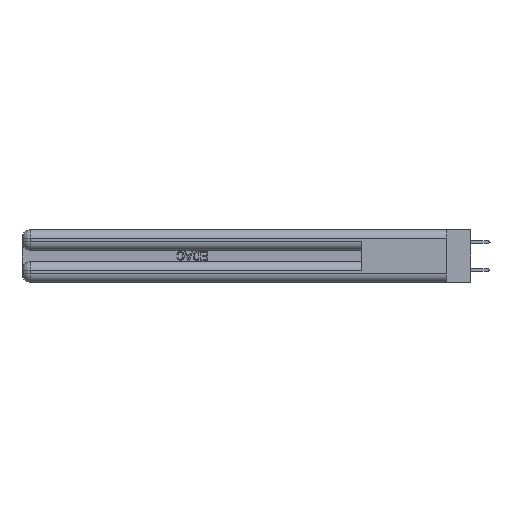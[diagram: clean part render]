
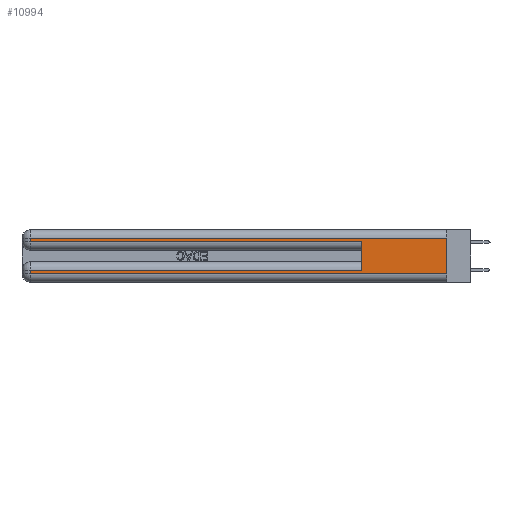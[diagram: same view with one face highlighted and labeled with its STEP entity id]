
A CAD part, left-side view. The second image highlights one B-rep face of the part: STEP entity #10994.
In plain terms, the highlighted planar face has unit normal (-1, 0, 0).
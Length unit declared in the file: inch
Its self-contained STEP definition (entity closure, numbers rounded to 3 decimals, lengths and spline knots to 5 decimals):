
#1044 = VERTEX_POINT ( 'NONE', #24151 ) ;
#1306 = CARTESIAN_POINT ( 'NONE',  ( 0., 0., 0.37 ) ) ;
#1368 = VECTOR ( 'NONE', #18233, 39.37008 ) ;
#1788 = CARTESIAN_POINT ( 'NONE',  ( 0., 2.94, 0.285 ) ) ;
#1818 = VERTEX_POINT ( 'NONE', #13859 ) ;
#2205 = EDGE_CURVE ( 'NONE', #2818, #11704, #24350, .T. ) ;
#2666 = CARTESIAN_POINT ( 'NONE',  ( 0., 0., 0.31 ) ) ;
#2701 = LINE ( 'NONE', #21302, #34925 ) ;
#2818 = VERTEX_POINT ( 'NONE', #1788 ) ;
#4094 = LINE ( 'NONE', #29023, #19522 ) ;
#4219 = CARTESIAN_POINT ( 'NONE',  ( 0., 0.6, 0.085 ) ) ;
#6178 = CARTESIAN_POINT ( 'NONE',  ( 0., 0., 0.06 ) ) ;
#6883 = CARTESIAN_POINT ( 'NONE',  ( 0., 0., 0.06 ) ) ;
#7442 = VECTOR ( 'NONE', #21534, 39.37008 ) ;
#7646 = VECTOR ( 'NONE', #18627, 39.37008 ) ;
#7894 = CARTESIAN_POINT ( 'NONE',  ( 0., 2.94, 0.06 ) ) ;
#7979 = EDGE_CURVE ( 'NONE', #14330, #1818, #37925, .T. ) ;
#8123 = CARTESIAN_POINT ( 'NONE',  ( 0., 0., 0.37 ) ) ;
#8813 = EDGE_CURVE ( 'NONE', #1818, #2818, #15207, .T. ) ;
#9780 = DIRECTION ( 'NONE',  ( 0., 1., 0. ) ) ;
#10994 = ADVANCED_FACE ( 'NONE', ( #35675 ), #36085, .F. ) ;
#11587 = ORIENTED_EDGE ( 'NONE', *, *, #7979, .T. ) ;
#11704 = VERTEX_POINT ( 'NONE', #35297 ) ;
#11729 = DIRECTION ( 'NONE',  ( 0., 1., 0. ) ) ;
#12151 = CARTESIAN_POINT ( 'NONE',  ( 0., 2.94, 0.37 ) ) ;
#12502 = EDGE_CURVE ( 'NONE', #14330, #17520, #14176, .T. ) ;
#12824 = EDGE_CURVE ( 'NONE', #32387, #17520, #24569, .T. ) ;
#13472 = LINE ( 'NONE', #29198, #18146 ) ;
#13502 = DIRECTION ( 'NONE',  ( 0., 0., -1. ) ) ;
#13506 = VECTOR ( 'NONE', #38465, 39.37008 ) ;
#13859 = CARTESIAN_POINT ( 'NONE',  ( 0., 2.94, 0.31 ) ) ;
#14176 = LINE ( 'NONE', #1306, #13506 ) ;
#14330 = VERTEX_POINT ( 'NONE', #2666 ) ;
#14664 = ORIENTED_EDGE ( 'NONE', *, *, #12824, .T. ) ;
#15207 = LINE ( 'NONE', #12151, #7442 ) ;
#15524 = EDGE_CURVE ( 'NONE', #1044, #32387, #4094, .T. ) ;
#16704 = DIRECTION ( 'NONE',  ( 0., 0., -1. ) ) ;
#17295 = ORIENTED_EDGE ( 'NONE', *, *, #15524, .T. ) ;
#17520 = VERTEX_POINT ( 'NONE', #6883 ) ;
#18146 = VECTOR ( 'NONE', #35299, 39.37008 ) ;
#18233 = DIRECTION ( 'NONE',  ( 0., -1., 0. ) ) ;
#18627 = DIRECTION ( 'NONE',  ( 0., -1., 0. ) ) ;
#19522 = VECTOR ( 'NONE', #13502, 39.37008 ) ;
#20545 = ORIENTED_EDGE ( 'NONE', *, *, #2205, .T. ) ;
#21302 = CARTESIAN_POINT ( 'NONE',  ( 0., 0., 0.085 ) ) ;
#21534 = DIRECTION ( 'NONE',  ( 0., 0., -1. ) ) ;
#24048 = ORIENTED_EDGE ( 'NONE', *, *, #12502, .F. ) ;
#24151 = CARTESIAN_POINT ( 'NONE',  ( 0., 2.94, 0.085 ) ) ;
#24350 = LINE ( 'NONE', #36796, #1368 ) ;
#24569 = LINE ( 'NONE', #6178, #7646 ) ;
#27483 = EDGE_CURVE ( 'NONE', #27990, #1044, #2701, .T. ) ;
#27990 = VERTEX_POINT ( 'NONE', #4219 ) ;
#29023 = CARTESIAN_POINT ( 'NONE',  ( 0., 2.94, 0.37 ) ) ;
#29198 = CARTESIAN_POINT ( 'NONE',  ( 0., 0.6, 0.145 ) ) ;
#30406 = EDGE_LOOP ( 'NONE', ( #24048, #11587, #31213, #20545, #34841, #36443, #17295, #14664 ) ) ;
#31213 = ORIENTED_EDGE ( 'NONE', *, *, #8813, .T. ) ;
#31885 = EDGE_CURVE ( 'NONE', #27990, #11704, #13472, .T. ) ;
#32220 = DIRECTION ( 'NONE',  ( 1., 0., 0. ) ) ;
#32387 = VERTEX_POINT ( 'NONE', #7894 ) ;
#34841 = ORIENTED_EDGE ( 'NONE', *, *, #31885, .F. ) ;
#34925 = VECTOR ( 'NONE', #11729, 39.37008 ) ;
#35297 = CARTESIAN_POINT ( 'NONE',  ( 0., 0.6, 0.285 ) ) ;
#35299 = DIRECTION ( 'NONE',  ( 0., 0., 1. ) ) ;
#35675 = FACE_OUTER_BOUND ( 'NONE', #30406, .T. ) ;
#36085 = PLANE ( 'NONE',  #40152 ) ;
#36443 = ORIENTED_EDGE ( 'NONE', *, *, #27483, .T. ) ;
#36796 = CARTESIAN_POINT ( 'NONE',  ( 0., 0., 0.285 ) ) ;
#36813 = VECTOR ( 'NONE', #9780, 39.37008 ) ;
#37730 = CARTESIAN_POINT ( 'NONE',  ( 0., 0., 0.31 ) ) ;
#37925 = LINE ( 'NONE', #37730, #36813 ) ;
#38465 = DIRECTION ( 'NONE',  ( 0., 0., -1. ) ) ;
#40152 = AXIS2_PLACEMENT_3D ( 'NONE', #8123, #32220, #16704 ) ;
